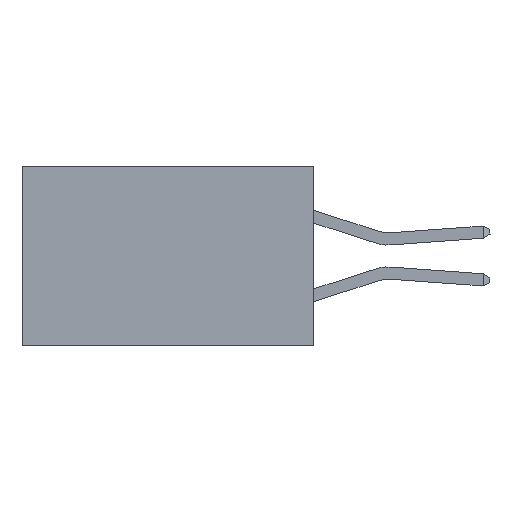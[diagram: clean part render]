
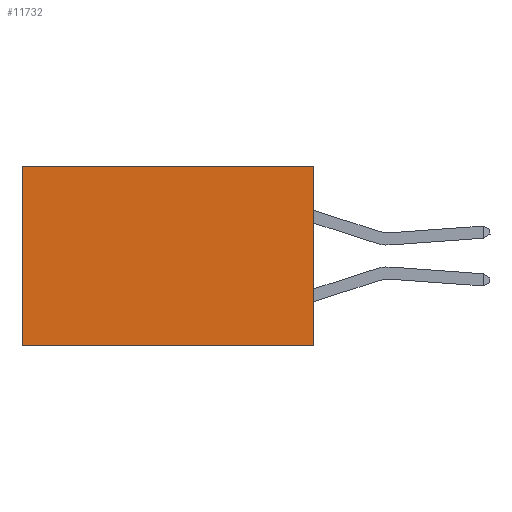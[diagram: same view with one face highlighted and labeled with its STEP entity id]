
A CAD part, left-side view. The second image highlights one B-rep face of the part: STEP entity #11732.
In plain terms, the highlighted planar face has unit normal (-1, 0, 0).
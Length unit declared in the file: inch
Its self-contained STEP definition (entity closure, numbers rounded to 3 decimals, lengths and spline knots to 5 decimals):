
#190 = VERTEX_POINT ( 'NONE', #11737 ) ;
#219 = VERTEX_POINT ( 'NONE', #9788 ) ;
#391 = FACE_OUTER_BOUND ( 'NONE', #5552, .T. ) ;
#1186 = ORIENTED_EDGE ( 'NONE', *, *, #5830, .F. ) ;
#1249 = VECTOR ( 'NONE', #5822, 39.37008 ) ;
#3096 = LINE ( 'NONE', #16649, #16458 ) ;
#4668 = DIRECTION ( 'NONE',  ( 0., 1., 0. ) ) ;
#5385 = LINE ( 'NONE', #12457, #21153 ) ;
#5552 = EDGE_LOOP ( 'NONE', ( #20453, #8958, #1186, #5944 ) ) ;
#5822 = DIRECTION ( 'NONE',  ( 0., 1., 0. ) ) ;
#5830 = EDGE_CURVE ( 'NONE', #190, #14539, #5385, .T. ) ;
#5944 = ORIENTED_EDGE ( 'NONE', *, *, #18430, .T. ) ;
#8958 = ORIENTED_EDGE ( 'NONE', *, *, #10224, .F. ) ;
#9788 = CARTESIAN_POINT ( 'NONE',  ( 0.2875, 0.6, -0.37 ) ) ;
#10224 = EDGE_CURVE ( 'NONE', #14539, #219, #11697, .T. ) ;
#10361 = PLANE ( 'NONE',  #17593 ) ;
#11697 = LINE ( 'NONE', #15846, #1249 ) ;
#11732 = ADVANCED_FACE ( 'NONE', ( #391 ), #10361, .F. ) ;
#11737 = CARTESIAN_POINT ( 'NONE',  ( 0.2875, 0., 0. ) ) ;
#12457 = CARTESIAN_POINT ( 'NONE',  ( 0.2875, 0., 0. ) ) ;
#14311 = DIRECTION ( 'NONE',  ( 0., 0., -1. ) ) ;
#14539 = VERTEX_POINT ( 'NONE', #18887 ) ;
#14889 = DIRECTION ( 'NONE',  ( 0., 0., -1. ) ) ;
#14974 = LINE ( 'NONE', #19465, #21288 ) ;
#15294 = CARTESIAN_POINT ( 'NONE',  ( 0.2875, 0.6, 0. ) ) ;
#15846 = CARTESIAN_POINT ( 'NONE',  ( 0.2875, 0., -0.37 ) ) ;
#16458 = VECTOR ( 'NONE', #4668, 39.37008 ) ;
#16649 = CARTESIAN_POINT ( 'NONE',  ( 0.2875, 0., 0. ) ) ;
#16697 = EDGE_CURVE ( 'NONE', #19318, #219, #14974, .T. ) ;
#17593 = AXIS2_PLACEMENT_3D ( 'NONE', #18224, #18810, #14889 ) ;
#17857 = DIRECTION ( 'NONE',  ( 0., 0., -1. ) ) ;
#18224 = CARTESIAN_POINT ( 'NONE',  ( 0.2875, 0., 0. ) ) ;
#18430 = EDGE_CURVE ( 'NONE', #190, #19318, #3096, .T. ) ;
#18810 = DIRECTION ( 'NONE',  ( 1., 0., 0. ) ) ;
#18887 = CARTESIAN_POINT ( 'NONE',  ( 0.2875, 0., -0.37 ) ) ;
#19318 = VERTEX_POINT ( 'NONE', #15294 ) ;
#19465 = CARTESIAN_POINT ( 'NONE',  ( 0.2875, 0.6, 0. ) ) ;
#20453 = ORIENTED_EDGE ( 'NONE', *, *, #16697, .T. ) ;
#21153 = VECTOR ( 'NONE', #14311, 39.37008 ) ;
#21288 = VECTOR ( 'NONE', #17857, 39.37008 ) ;
